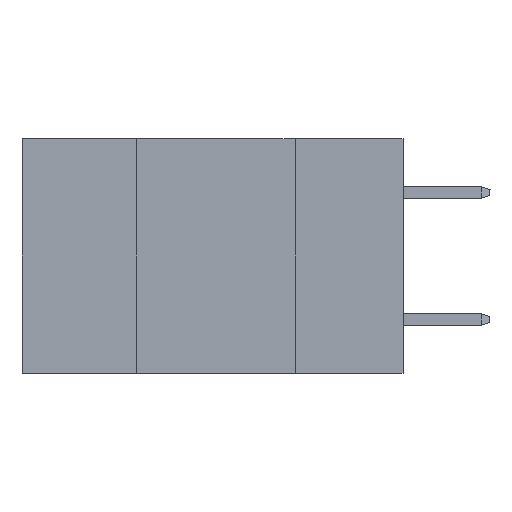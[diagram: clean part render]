
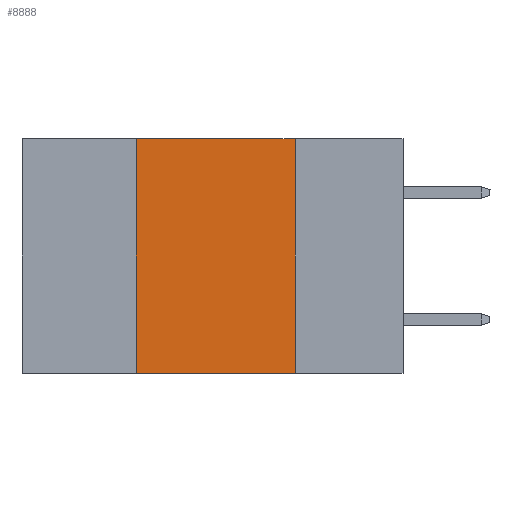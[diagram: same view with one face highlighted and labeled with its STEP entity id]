
A CAD part, left-side view. The second image highlights one B-rep face of the part: STEP entity #8888.
In plain terms, the highlighted planar face has unit normal (-1, 0, 0).
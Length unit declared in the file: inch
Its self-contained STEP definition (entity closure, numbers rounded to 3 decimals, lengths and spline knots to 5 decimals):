
#1042 = EDGE_CURVE ( 'NONE', #5500, #6588, #16352, .T. ) ;
#1858 = ORIENTED_EDGE ( 'NONE', *, *, #1042, .T. ) ;
#2482 = DIRECTION ( 'NONE',  ( 0., 0., -1. ) ) ;
#2970 = CARTESIAN_POINT ( 'NONE',  ( 0., 0.6, -0.37 ) ) ;
#3069 = DIRECTION ( 'NONE',  ( 0., -1., 0. ) ) ;
#3187 = EDGE_CURVE ( 'NONE', #5500, #5890, #10334, .T. ) ;
#5038 = CARTESIAN_POINT ( 'NONE',  ( 0., 0.17, 0. ) ) ;
#5091 = VERTEX_POINT ( 'NONE', #5038 ) ;
#5500 = VERTEX_POINT ( 'NONE', #11493 ) ;
#5511 = EDGE_CURVE ( 'NONE', #5890, #5091, #8405, .T. ) ;
#5890 = VERTEX_POINT ( 'NONE', #14072 ) ;
#6588 = VERTEX_POINT ( 'NONE', #13784 ) ;
#6871 = EDGE_CURVE ( 'NONE', #5091, #6588, #12313, .T. ) ;
#7283 = VECTOR ( 'NONE', #16990, 39.37008 ) ;
#7692 = DIRECTION ( 'NONE',  ( 0., 0., -1. ) ) ;
#8405 = LINE ( 'NONE', #10327, #19260 ) ;
#8638 = CARTESIAN_POINT ( 'NONE',  ( 0., 0.42, 0. ) ) ;
#8888 = ADVANCED_FACE ( 'NONE', ( #14310 ), #15974, .F. ) ;
#9797 = VECTOR ( 'NONE', #3069, 39.37008 ) ;
#10327 = CARTESIAN_POINT ( 'NONE',  ( 0., 0.6, 0. ) ) ;
#10334 = LINE ( 'NONE', #8638, #7283 ) ;
#10621 = CARTESIAN_POINT ( 'NONE',  ( 0., 0.17, 0. ) ) ;
#10746 = CARTESIAN_POINT ( 'NONE',  ( 0., 0.6, 0. ) ) ;
#10761 = ORIENTED_EDGE ( 'NONE', *, *, #3187, .F. ) ;
#11493 = CARTESIAN_POINT ( 'NONE',  ( 0., 0.42, -0.37 ) ) ;
#12313 = LINE ( 'NONE', #10621, #16456 ) ;
#13784 = CARTESIAN_POINT ( 'NONE',  ( 0., 0.17, -0.37 ) ) ;
#14072 = CARTESIAN_POINT ( 'NONE',  ( 0., 0.42, 0. ) ) ;
#14310 = FACE_OUTER_BOUND ( 'NONE', #18728, .T. ) ;
#15974 = PLANE ( 'NONE',  #17913 ) ;
#16352 = LINE ( 'NONE', #2970, #9797 ) ;
#16456 = VECTOR ( 'NONE', #7692, 39.37008 ) ;
#16984 = DIRECTION ( 'NONE',  ( 0., -1., 0. ) ) ;
#16990 = DIRECTION ( 'NONE',  ( 0., 0., 1. ) ) ;
#17392 = DIRECTION ( 'NONE',  ( 1., 0., 0. ) ) ;
#17913 = AXIS2_PLACEMENT_3D ( 'NONE', #10746, #17392, #2482 ) ;
#18465 = ORIENTED_EDGE ( 'NONE', *, *, #6871, .F. ) ;
#18728 = EDGE_LOOP ( 'NONE', ( #18465, #20338, #10761, #1858 ) ) ;
#19260 = VECTOR ( 'NONE', #16984, 39.37008 ) ;
#20338 = ORIENTED_EDGE ( 'NONE', *, *, #5511, .F. ) ;
